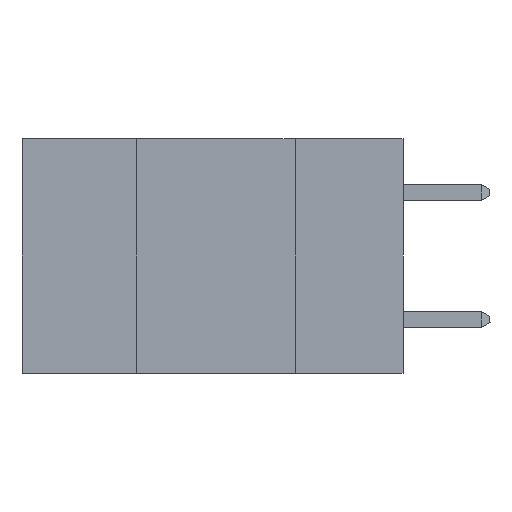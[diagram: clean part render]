
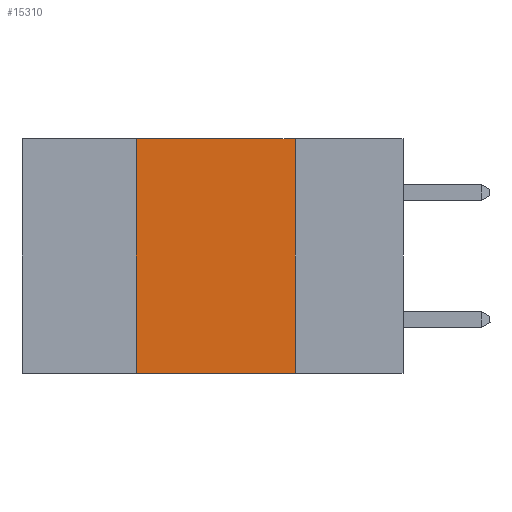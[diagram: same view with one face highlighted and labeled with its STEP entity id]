
A CAD part, left-side view. The second image highlights one B-rep face of the part: STEP entity #15310.
In plain terms, the highlighted planar face has unit normal (-1, 0, 0).
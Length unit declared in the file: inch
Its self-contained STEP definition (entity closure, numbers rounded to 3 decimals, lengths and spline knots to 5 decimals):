
#686 = LINE ( 'NONE', #3849, #1223 ) ;
#704 = CARTESIAN_POINT ( 'NONE',  ( 0., 0.6, -0.37 ) ) ;
#1223 = VECTOR ( 'NONE', #5622, 39.37008 ) ;
#1412 = ORIENTED_EDGE ( 'NONE', *, *, #7505, .F. ) ;
#1454 = VERTEX_POINT ( 'NONE', #4373 ) ;
#1499 = LINE ( 'NONE', #704, #5617 ) ;
#2088 = CARTESIAN_POINT ( 'NONE',  ( 0., 0.6, 0. ) ) ;
#2558 = ORIENTED_EDGE ( 'NONE', *, *, #8566, .F. ) ;
#3837 = DIRECTION ( 'NONE',  ( 1., 0., 0. ) ) ;
#3849 = CARTESIAN_POINT ( 'NONE',  ( 0., 0.42, 0. ) ) ;
#4002 = ORIENTED_EDGE ( 'NONE', *, *, #10668, .F. ) ;
#4373 = CARTESIAN_POINT ( 'NONE',  ( 0., 0.42, -0.37 ) ) ;
#4497 = EDGE_LOOP ( 'NONE', ( #4002, #2558, #1412, #16816 ) ) ;
#4788 = FACE_OUTER_BOUND ( 'NONE', #4497, .T. ) ;
#5109 = CARTESIAN_POINT ( 'NONE',  ( 0., 0.6, 0. ) ) ;
#5433 = CARTESIAN_POINT ( 'NONE',  ( 0., 0.17, 0. ) ) ;
#5560 = LINE ( 'NONE', #5109, #6100 ) ;
#5617 = VECTOR ( 'NONE', #16046, 39.37008 ) ;
#5622 = DIRECTION ( 'NONE',  ( 0., 0., 1. ) ) ;
#5859 = DIRECTION ( 'NONE',  ( 0., 0., -1. ) ) ;
#6100 = VECTOR ( 'NONE', #20227, 39.37008 ) ;
#7505 = EDGE_CURVE ( 'NONE', #1454, #12300, #686, .T. ) ;
#8566 = EDGE_CURVE ( 'NONE', #12300, #21462, #5560, .T. ) ;
#10668 = EDGE_CURVE ( 'NONE', #21462, #15328, #13666, .T. ) ;
#12300 = VERTEX_POINT ( 'NONE', #19127 ) ;
#12344 = PLANE ( 'NONE',  #21173 ) ;
#13666 = LINE ( 'NONE', #14253, #17579 ) ;
#14253 = CARTESIAN_POINT ( 'NONE',  ( 0., 0.17, 0. ) ) ;
#15310 = ADVANCED_FACE ( 'NONE', ( #4788 ), #12344, .F. ) ;
#15328 = VERTEX_POINT ( 'NONE', #19094 ) ;
#15471 = EDGE_CURVE ( 'NONE', #1454, #15328, #1499, .T. ) ;
#15684 = DIRECTION ( 'NONE',  ( 0., 0., -1. ) ) ;
#16046 = DIRECTION ( 'NONE',  ( 0., -1., 0. ) ) ;
#16816 = ORIENTED_EDGE ( 'NONE', *, *, #15471, .T. ) ;
#17579 = VECTOR ( 'NONE', #5859, 39.37008 ) ;
#19094 = CARTESIAN_POINT ( 'NONE',  ( 0., 0.17, -0.37 ) ) ;
#19127 = CARTESIAN_POINT ( 'NONE',  ( 0., 0.42, 0. ) ) ;
#20227 = DIRECTION ( 'NONE',  ( 0., -1., 0. ) ) ;
#21173 = AXIS2_PLACEMENT_3D ( 'NONE', #2088, #3837, #15684 ) ;
#21462 = VERTEX_POINT ( 'NONE', #5433 ) ;
